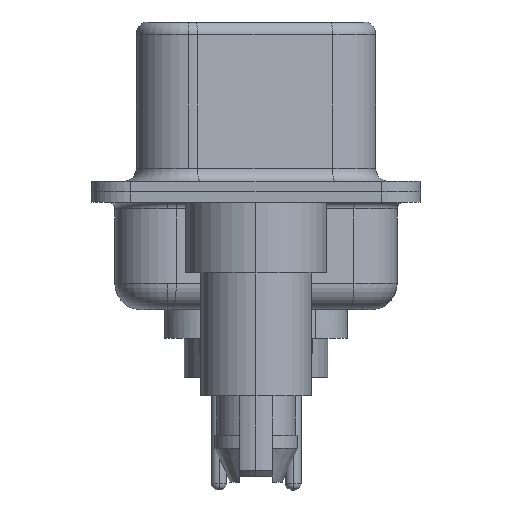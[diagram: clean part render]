
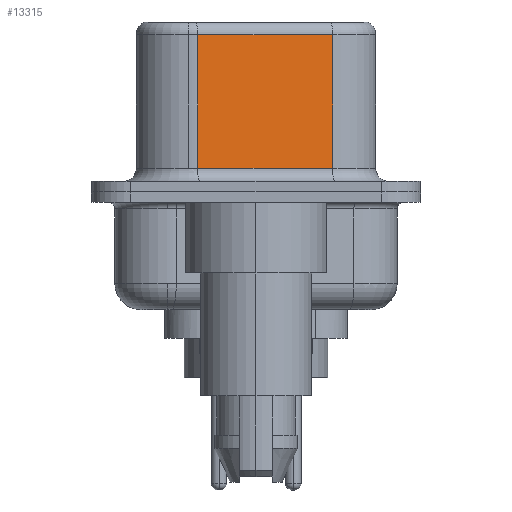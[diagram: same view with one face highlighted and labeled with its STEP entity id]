
A CAD part, left-side view. The second image highlights one B-rep face of the part: STEP entity #13315.
In plain terms, the highlighted planar face has unit normal (-0.985, -0.174, 0).
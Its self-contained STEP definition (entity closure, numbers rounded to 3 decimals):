
#481 = CARTESIAN_POINT ( 'NONE',  ( 4.565, -2.927, 0.9 ) ) ;
#960 = CARTESIAN_POINT ( 'NONE',  ( 3.655, 2.233, 6.02 ) ) ;
#977 = AXIS2_PLACEMENT_3D ( 'NONE', #10414, #7668, #17430 ) ;
#1212 = EDGE_LOOP ( 'NONE', ( #5790, #14327, #14101, #5633 ) ) ;
#1568 = VERTEX_POINT ( 'NONE', #960 ) ;
#1935 = VERTEX_POINT ( 'NONE', #2604 ) ;
#1958 = LINE ( 'NONE', #13613, #12249 ) ;
#2429 = DIRECTION ( 'NONE',  ( 0., 0., -1. ) ) ;
#2604 = CARTESIAN_POINT ( 'NONE',  ( 3.655, 2.233, 0.9 ) ) ;
#3943 = DIRECTION ( 'NONE',  ( 0.174, -0.985, 0. ) ) ;
#5613 = CARTESIAN_POINT ( 'NONE',  ( 4.565, -2.927, 6.02 ) ) ;
#5633 = ORIENTED_EDGE ( 'NONE', *, *, #9542, .T. ) ;
#5790 = ORIENTED_EDGE ( 'NONE', *, *, #8823, .F. ) ;
#5997 = EDGE_CURVE ( 'NONE', #14129, #1568, #14839, .T. ) ;
#6151 = VECTOR ( 'NONE', #11599, 1000. ) ;
#6591 = LINE ( 'NONE', #12967, #6151 ) ;
#7668 = DIRECTION ( 'NONE',  ( 0.985, 0.174, 0. ) ) ;
#8823 = EDGE_CURVE ( 'NONE', #14129, #18007, #1958, .T. ) ;
#9542 = EDGE_CURVE ( 'NONE', #1935, #18007, #15753, .T. ) ;
#9979 = DIRECTION ( 'NONE',  ( -0.174, 0.985, 0. ) ) ;
#10414 = CARTESIAN_POINT ( 'NONE',  ( 4.565, -2.927, 6.52 ) ) ;
#11124 = VECTOR ( 'NONE', #9979, 1000. ) ;
#11599 = DIRECTION ( 'NONE',  ( 0., 0., -1. ) ) ;
#12249 = VECTOR ( 'NONE', #2429, 1000. ) ;
#12273 = CARTESIAN_POINT ( 'NONE',  ( 4.565, -2.927, 6.02 ) ) ;
#12810 = EDGE_CURVE ( 'NONE', #1568, #1935, #6591, .T. ) ;
#12967 = CARTESIAN_POINT ( 'NONE',  ( 3.655, 2.233, 6.52 ) ) ;
#13160 = PLANE ( 'NONE',  #977 ) ;
#13315 = ADVANCED_FACE ( 'NONE', ( #15865 ), #13160, .F. ) ;
#13613 = CARTESIAN_POINT ( 'NONE',  ( 4.565, -2.927, 6.52 ) ) ;
#14101 = ORIENTED_EDGE ( 'NONE', *, *, #12810, .T. ) ;
#14129 = VERTEX_POINT ( 'NONE', #5613 ) ;
#14327 = ORIENTED_EDGE ( 'NONE', *, *, #5997, .T. ) ;
#14839 = LINE ( 'NONE', #12273, #11124 ) ;
#15753 = LINE ( 'NONE', #17855, #16195 ) ;
#15865 = FACE_OUTER_BOUND ( 'NONE', #1212, .T. ) ;
#16195 = VECTOR ( 'NONE', #3943, 1000. ) ;
#17430 = DIRECTION ( 'NONE',  ( -0.174, 0.985, 0. ) ) ;
#17855 = CARTESIAN_POINT ( 'NONE',  ( 4.565, -2.927, 0.9 ) ) ;
#18007 = VERTEX_POINT ( 'NONE', #481 ) ;
